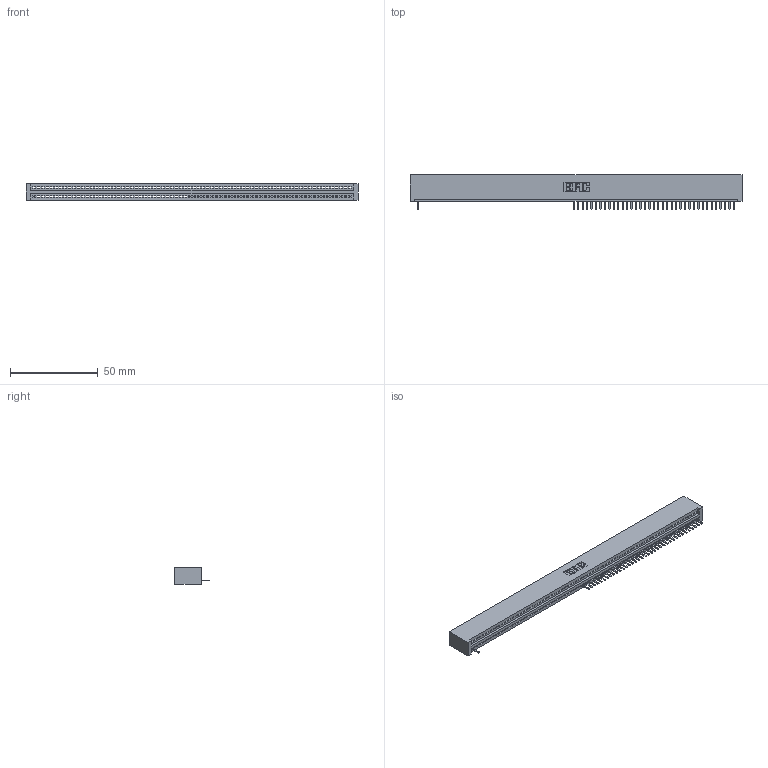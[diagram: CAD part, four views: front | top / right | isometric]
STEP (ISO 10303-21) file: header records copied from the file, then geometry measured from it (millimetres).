
FILE_DESCRIPTION (( 'STEP AP203' ), '1' );
FILE_NAME ('395-072-520-101.STEP', '2018-11-27T07:45:34', ( '' ), ( '' ), 'SwSTEP 2.0', 'SolidWorks 2016', '' );
FILE_SCHEMA (( 'CONFIG_CONTROL_DESIGN' ));
Length unit declared in the file: inch
Products named in the file (3): 395-072-520-101; 345 Part_No Mounting Lugs; 345-292-001_345-293-120
Assembly tree (39 placements, depth 2):
  395-072-520-101
    345 Part_No Mounting Lugs
    345-292-001_345-293-120  x38
Bounding box: 189.48 x 19.68 x 9.4 mm (x, y, z)
Volume: 18328.9 mm3; surface area: 22530.1 mm2
Topology: 39 solids, 39 shells, 3018 faces, 9145 edges, 5994 vertices
Faces by surface type: plane 2148, cylinder 870
Entity records: 48899 total; most frequent: ORIENTED_EDGE 8670, CARTESIAN_POINT 8642, DIRECTION 7447, EDGE_CURVE 4335, LINE 3919, VECTOR 3919, VERTEX_POINT 2886, AXIS2_PLACEMENT_3D 1764
